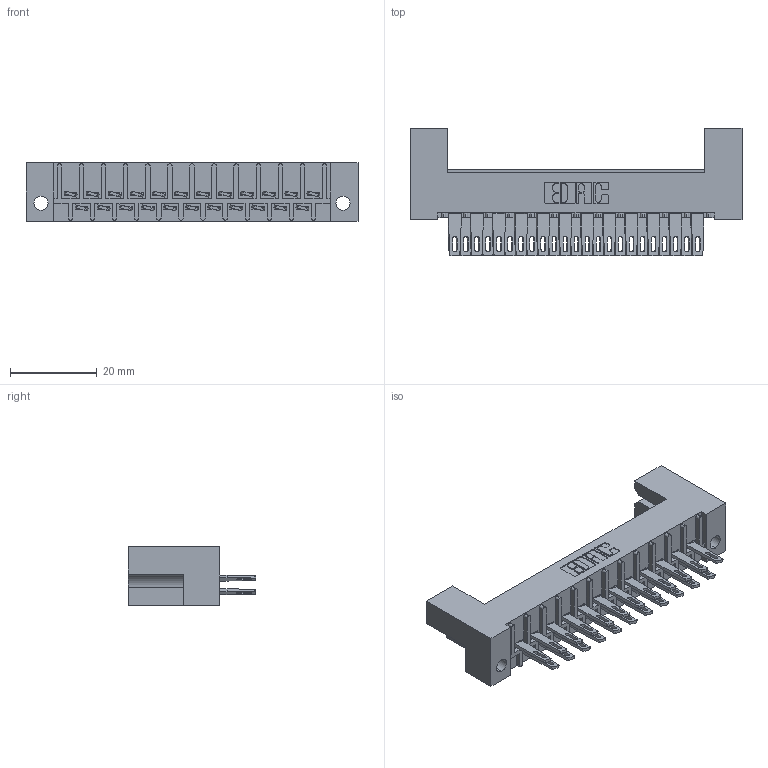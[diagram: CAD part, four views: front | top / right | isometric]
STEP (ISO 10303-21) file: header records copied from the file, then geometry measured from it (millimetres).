
FILE_DESCRIPTION (( 'STEP AP203' ), '1' );
FILE_NAME ('408-023-500-222.STEP', '2019-11-04T18:41:07', ( '' ), ( '' ), 'SwSTEP 2.0', 'SolidWorks 2016', '' );
FILE_SCHEMA (( 'CONFIG_CONTROL_DESIGN' ));
Length unit declared in the file: inch
Products named in the file (3): 408-023-500-222; 408-290-001_408-290-100; 408 Part_023 - 2
Assembly tree (24 placements, depth 2):
  408-023-500-222
    408 Part_023 - 2
    408-290-001_408-290-100  x23
Bounding box: 76.35 x 29.31 x 13.49 mm (x, y, z)
Volume: 10150.8 mm3; surface area: 11843.9 mm2
Topology: 24 solids, 24 shells, 1450 faces, 4000 edges, 2604 vertices
Faces by surface type: plane 1032, cylinder 326, bspline 92
Entity records: 19835 total; most frequent: CARTESIAN_POINT 3429, ORIENTED_EDGE 3336, DIRECTION 3058, EDGE_CURVE 1668, VECTOR 1456, LINE 1456, VERTEX_POINT 1108, AXIS2_PLACEMENT_3D 801
